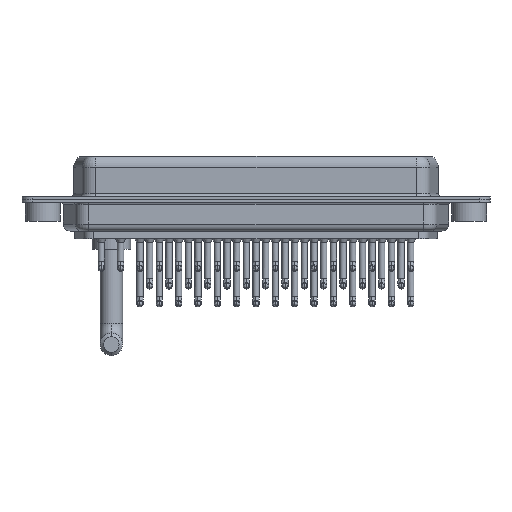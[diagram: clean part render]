
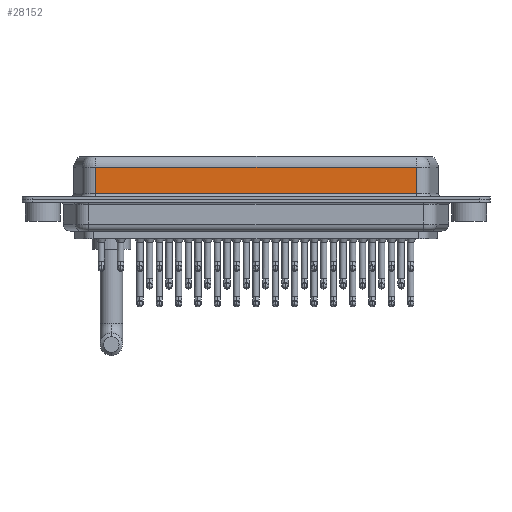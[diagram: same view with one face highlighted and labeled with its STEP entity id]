
A CAD part, front view. The second image highlights one B-rep face of the part: STEP entity #28152.
In plain terms, the highlighted planar face has unit normal (0, -1, 0).
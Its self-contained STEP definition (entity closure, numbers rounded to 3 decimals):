
#99 = VECTOR ( 'NONE', #32937, 1000. ) ;
#1936 = LINE ( 'NONE', #22875, #16997 ) ;
#2344 = CARTESIAN_POINT ( 'NONE',  ( 53.41, -5.375, 4.65 ) ) ;
#2718 = EDGE_CURVE ( 'NONE', #6738, #11410, #1936, .T. ) ;
#4696 = EDGE_CURVE ( 'NONE', #20371, #26745, #14651, .T. ) ;
#4840 = ORIENTED_EDGE ( 'NONE', *, *, #2718, .T. ) ;
#4938 = VECTOR ( 'NONE', #16059, 1000. ) ;
#4986 = DIRECTION ( 'NONE',  ( 1., 0., 0. ) ) ;
#6286 = ORIENTED_EDGE ( 'NONE', *, *, #30711, .F. ) ;
#6738 = VERTEX_POINT ( 'NONE', #17122 ) ;
#7808 = FACE_OUTER_BOUND ( 'NONE', #33489, .T. ) ;
#9345 = AXIS2_PLACEMENT_3D ( 'NONE', #18298, #15723, #28435 ) ;
#11410 = VERTEX_POINT ( 'NONE', #32293 ) ;
#13829 = CARTESIAN_POINT ( 'NONE',  ( 7.59, -5.375, 6.4 ) ) ;
#14443 = ORIENTED_EDGE ( 'NONE', *, *, #4696, .T. ) ;
#14651 = LINE ( 'NONE', #25133, #28090 ) ;
#15723 = DIRECTION ( 'NONE',  ( 0., 1., 0. ) ) ;
#16059 = DIRECTION ( 'NONE',  ( 0., 0., -1. ) ) ;
#16092 = CARTESIAN_POINT ( 'NONE',  ( 7.59, -5.375, 4.65 ) ) ;
#16997 = VECTOR ( 'NONE', #4986, 1000. ) ;
#17122 = CARTESIAN_POINT ( 'NONE',  ( 7.59, -5.375, 0.9 ) ) ;
#17386 = DIRECTION ( 'NONE',  ( -1., 0., 0. ) ) ;
#18020 = ORIENTED_EDGE ( 'NONE', *, *, #29515, .T. ) ;
#18298 = CARTESIAN_POINT ( 'NONE',  ( 53.41, -5.375, 6.4 ) ) ;
#19214 = LINE ( 'NONE', #32431, #99 ) ;
#20371 = VERTEX_POINT ( 'NONE', #2344 ) ;
#22875 = CARTESIAN_POINT ( 'NONE',  ( 53.41, -5.375, 0.9 ) ) ;
#25133 = CARTESIAN_POINT ( 'NONE',  ( 53.41, -5.375, 4.65 ) ) ;
#25538 = PLANE ( 'NONE',  #9345 ) ;
#26745 = VERTEX_POINT ( 'NONE', #16092 ) ;
#28090 = VECTOR ( 'NONE', #17386, 1000. ) ;
#28152 = ADVANCED_FACE ( 'NONE', ( #7808 ), #25538, .F. ) ;
#28435 = DIRECTION ( 'NONE',  ( 0., 0., 1. ) ) ;
#29515 = EDGE_CURVE ( 'NONE', #26745, #6738, #29632, .T. ) ;
#29632 = LINE ( 'NONE', #13829, #4938 ) ;
#30711 = EDGE_CURVE ( 'NONE', #20371, #11410, #19214, .T. ) ;
#32293 = CARTESIAN_POINT ( 'NONE',  ( 53.41, -5.375, 0.9 ) ) ;
#32431 = CARTESIAN_POINT ( 'NONE',  ( 53.41, -5.375, 6.4 ) ) ;
#32937 = DIRECTION ( 'NONE',  ( 0., 0., -1. ) ) ;
#33489 = EDGE_LOOP ( 'NONE', ( #6286, #14443, #18020, #4840 ) ) ;
